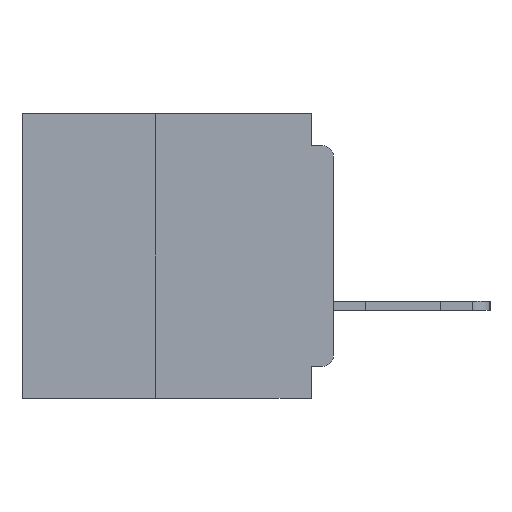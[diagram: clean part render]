
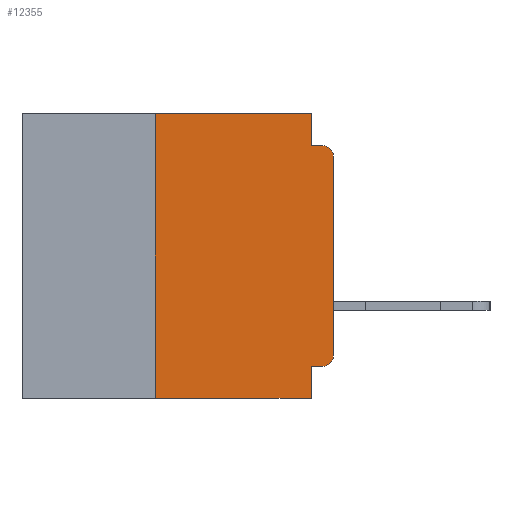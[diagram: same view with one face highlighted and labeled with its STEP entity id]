
A CAD part, left-side view. The second image highlights one B-rep face of the part: STEP entity #12355.
In plain terms, the highlighted planar face has unit normal (-1, 0, 0).
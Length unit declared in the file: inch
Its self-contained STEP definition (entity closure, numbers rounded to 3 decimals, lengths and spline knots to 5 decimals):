
#372 = CARTESIAN_POINT ( 'NONE',  ( 0., 0., 0. ) ) ;
#1070 = CARTESIAN_POINT ( 'NONE',  ( 0., 0.015, -0.045 ) ) ;
#2979 = CARTESIAN_POINT ( 'NONE',  ( 0., 0.437, 0. ) ) ;
#3573 = CARTESIAN_POINT ( 'NONE',  ( 0., 0.015, -0.355 ) ) ;
#3980 = CARTESIAN_POINT ( 'NONE',  ( 0., 0.031, -0.045 ) ) ;
#8225 = CARTESIAN_POINT ( 'NONE',  ( 0., 0.25, -0.4 ) ) ;
#10084 = EDGE_CURVE ( 'NONE', #27166, #14799, #32689, .T. ) ;
#10406 = VERTEX_POINT ( 'NONE', #1070 ) ;
#10827 = ORIENTED_EDGE ( 'NONE', *, *, #16006, .T. ) ;
#11681 = VECTOR ( 'NONE', #49993, 39.37008 ) ;
#11961 = EDGE_CURVE ( 'NONE', #42572, #14564, #48139, .T. ) ;
#12188 = DIRECTION ( 'NONE',  ( 1., 0., 0. ) ) ;
#12355 = ADVANCED_FACE ( 'NONE', ( #25286 ), #48567, .F. ) ;
#12439 = EDGE_CURVE ( 'NONE', #44877, #45867, #45222, .T. ) ;
#12743 = VERTEX_POINT ( 'NONE', #46924 ) ;
#13738 = ORIENTED_EDGE ( 'NONE', *, *, #10084, .F. ) ;
#14188 = CARTESIAN_POINT ( 'NONE',  ( 0., 0.015, -0.06 ) ) ;
#14564 = VERTEX_POINT ( 'NONE', #3980 ) ;
#14688 = ORIENTED_EDGE ( 'NONE', *, *, #23190, .T. ) ;
#14799 = VERTEX_POINT ( 'NONE', #24204 ) ;
#16006 = EDGE_CURVE ( 'NONE', #40195, #10406, #35713, .T. ) ;
#18722 = DIRECTION ( 'NONE',  ( -1., 0., 0. ) ) ;
#18772 = EDGE_CURVE ( 'NONE', #44877, #14799, #38302, .T. ) ;
#18813 = DIRECTION ( 'NONE',  ( 0., 0., -1. ) ) ;
#19848 = DIRECTION ( 'NONE',  ( 0., -1., 0. ) ) ;
#21705 = EDGE_CURVE ( 'NONE', #27004, #27166, #53236, .T. ) ;
#21904 = DIRECTION ( 'NONE',  ( 0., -1., 0. ) ) ;
#22003 = VECTOR ( 'NONE', #21904, 39.37008 ) ;
#22034 = DIRECTION ( 'NONE',  ( 0., 0., 1. ) ) ;
#22400 = CARTESIAN_POINT ( 'NONE',  ( 0., 0.25, -0.4 ) ) ;
#22733 = CARTESIAN_POINT ( 'NONE',  ( 0., 0., -0.06 ) ) ;
#22753 = AXIS2_PLACEMENT_3D ( 'NONE', #2979, #12188, #44182 ) ;
#23190 = EDGE_CURVE ( 'NONE', #27004, #12743, #52321, .T. ) ;
#23706 = ORIENTED_EDGE ( 'NONE', *, *, #21705, .F. ) ;
#24204 = CARTESIAN_POINT ( 'NONE',  ( 0., 0.031, -0.4 ) ) ;
#24747 = VECTOR ( 'NONE', #55818, 39.37008 ) ;
#25286 = FACE_OUTER_BOUND ( 'NONE', #56799, .T. ) ;
#25980 = DIRECTION ( 'NONE',  ( 0., 1., 0. ) ) ;
#26424 = EDGE_CURVE ( 'NONE', #14564, #10406, #46237, .T. ) ;
#27004 = VERTEX_POINT ( 'NONE', #3573 ) ;
#27166 = VERTEX_POINT ( 'NONE', #45918 ) ;
#27218 = ORIENTED_EDGE ( 'NONE', *, *, #52986, .T. ) ;
#31210 = LINE ( 'NONE', #372, #41921 ) ;
#31338 = ORIENTED_EDGE ( 'NONE', *, *, #26424, .F. ) ;
#31787 = CARTESIAN_POINT ( 'NONE',  ( 0., 0.25, 0. ) ) ;
#32689 = LINE ( 'NONE', #49130, #52587 ) ;
#34483 = LINE ( 'NONE', #56112, #43733 ) ;
#34990 = ORIENTED_EDGE ( 'NONE', *, *, #11961, .F. ) ;
#35713 = CIRCLE ( 'NONE', #58777, 0.015 ) ;
#38302 = LINE ( 'NONE', #51239, #24747 ) ;
#40195 = VERTEX_POINT ( 'NONE', #22733 ) ;
#41085 = CARTESIAN_POINT ( 'NONE',  ( 0., 0.031, 0. ) ) ;
#41199 = VECTOR ( 'NONE', #25980, 39.37008 ) ;
#41696 = DIRECTION ( 'NONE',  ( 0., 0., 1. ) ) ;
#41921 = VECTOR ( 'NONE', #41696, 39.37008 ) ;
#42572 = VERTEX_POINT ( 'NONE', #50719 ) ;
#43733 = VECTOR ( 'NONE', #19848, 39.37008 ) ;
#43816 = VECTOR ( 'NONE', #22034, 39.37008 ) ;
#44092 = CARTESIAN_POINT ( 'NONE',  ( 0., 0., -0.355 ) ) ;
#44182 = DIRECTION ( 'NONE',  ( 0., 0., -1. ) ) ;
#44877 = VERTEX_POINT ( 'NONE', #22400 ) ;
#45222 = LINE ( 'NONE', #8225, #43816 ) ;
#45867 = VERTEX_POINT ( 'NONE', #31787 ) ;
#45918 = CARTESIAN_POINT ( 'NONE',  ( 0., 0.031, -0.355 ) ) ;
#46077 = CARTESIAN_POINT ( 'NONE',  ( 0., 0.015, -0.34 ) ) ;
#46157 = DIRECTION ( 'NONE',  ( -1., 0., 0. ) ) ;
#46237 = LINE ( 'NONE', #58342, #22003 ) ;
#46924 = CARTESIAN_POINT ( 'NONE',  ( 0., 0., -0.34 ) ) ;
#47625 = ORIENTED_EDGE ( 'NONE', *, *, #12439, .F. ) ;
#48139 = LINE ( 'NONE', #41085, #11681 ) ;
#48567 = PLANE ( 'NONE',  #22753 ) ;
#49130 = CARTESIAN_POINT ( 'NONE',  ( 0., 0.031, -0.4 ) ) ;
#49993 = DIRECTION ( 'NONE',  ( 0., 0., -1. ) ) ;
#50633 = DIRECTION ( 'NONE',  ( 0., 0., -1. ) ) ;
#50719 = CARTESIAN_POINT ( 'NONE',  ( 0., 0.031, 0. ) ) ;
#51239 = CARTESIAN_POINT ( 'NONE',  ( 0., 0.437, -0.4 ) ) ;
#52321 = CIRCLE ( 'NONE', #57893, 0.015 ) ;
#52587 = VECTOR ( 'NONE', #58077, 39.37008 ) ;
#52986 = EDGE_CURVE ( 'NONE', #12743, #40195, #31210, .T. ) ;
#53236 = LINE ( 'NONE', #44092, #41199 ) ;
#55273 = EDGE_CURVE ( 'NONE', #45867, #42572, #34483, .T. ) ;
#55280 = ORIENTED_EDGE ( 'NONE', *, *, #55273, .F. ) ;
#55818 = DIRECTION ( 'NONE',  ( 0., -1., 0. ) ) ;
#56112 = CARTESIAN_POINT ( 'NONE',  ( 0., 0.437, 0. ) ) ;
#56799 = EDGE_LOOP ( 'NONE', ( #27218, #10827, #31338, #34990, #55280, #47625, #59196, #13738, #23706, #14688 ) ) ;
#57893 = AXIS2_PLACEMENT_3D ( 'NONE', #46077, #18722, #50633 ) ;
#58077 = DIRECTION ( 'NONE',  ( 0., 0., -1. ) ) ;
#58342 = CARTESIAN_POINT ( 'NONE',  ( 0., 0., -0.045 ) ) ;
#58777 = AXIS2_PLACEMENT_3D ( 'NONE', #14188, #46157, #18813 ) ;
#59196 = ORIENTED_EDGE ( 'NONE', *, *, #18772, .T. ) ;
